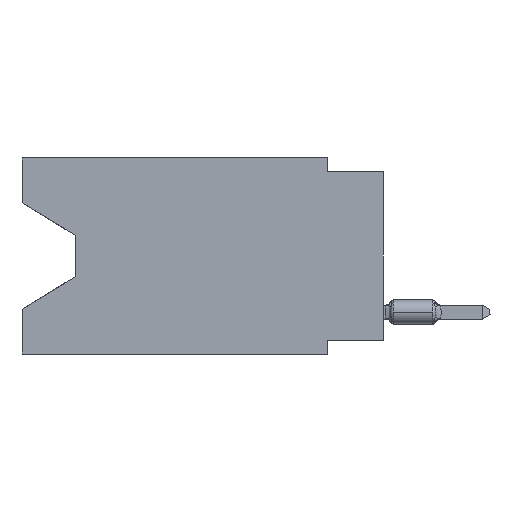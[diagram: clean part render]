
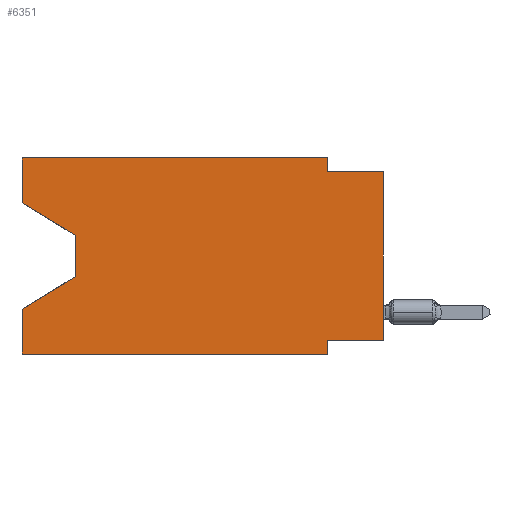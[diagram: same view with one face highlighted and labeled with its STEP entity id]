
A CAD part, left-side view. The second image highlights one B-rep face of the part: STEP entity #6351.
In plain terms, the highlighted planar face has unit normal (-1, 0, 0).
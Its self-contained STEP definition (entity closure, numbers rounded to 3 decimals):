
#263 = ORIENTED_EDGE ( 'NONE', *, *, #25929, .F. ) ;
#275 = CARTESIAN_POINT ( 'NONE',  ( 0., 0., -0.635 ) ) ;
#496 = ORIENTED_EDGE ( 'NONE', *, *, #4516, .T. ) ;
#847 = DIRECTION ( 'NONE',  ( 0., 0., -1. ) ) ;
#1204 = VERTEX_POINT ( 'NONE', #7517 ) ;
#1398 = EDGE_CURVE ( 'NONE', #16538, #1204, #17957, .T. ) ;
#1582 = EDGE_CURVE ( 'NONE', #8693, #20321, #19300, .T. ) ;
#1732 = ORIENTED_EDGE ( 'NONE', *, *, #1398, .F. ) ;
#1994 = EDGE_CURVE ( 'NONE', #21715, #24187, #12815, .T. ) ;
#2340 = CARTESIAN_POINT ( 'NONE',  ( 0., 16.383, 0. ) ) ;
#2963 = VECTOR ( 'NONE', #21807, 1000. ) ;
#3380 = VECTOR ( 'NONE', #6443, 1000. ) ;
#3395 = ORIENTED_EDGE ( 'NONE', *, *, #23280, .T. ) ;
#3563 = VECTOR ( 'NONE', #15848, 1000. ) ;
#3915 = VERTEX_POINT ( 'NONE', #27384 ) ;
#4516 = EDGE_CURVE ( 'NONE', #3915, #8952, #26525, .T. ) ;
#4691 = VECTOR ( 'NONE', #10370, 1000. ) ;
#4706 = VECTOR ( 'NONE', #27392, 1000. ) ;
#4714 = CARTESIAN_POINT ( 'NONE',  ( 0., 16.383, -6.852 ) ) ;
#5700 = ORIENTED_EDGE ( 'NONE', *, *, #8564, .F. ) ;
#5743 = EDGE_CURVE ( 'NONE', #1204, #20321, #18812, .T. ) ;
#6062 = DIRECTION ( 'NONE',  ( 1., 0., 0. ) ) ;
#6351 = ADVANCED_FACE ( 'NONE', ( #15439 ), #19857, .F. ) ;
#6443 = DIRECTION ( 'NONE',  ( 0., 1., 0. ) ) ;
#7517 = CARTESIAN_POINT ( 'NONE',  ( 0., 2.54, -8.255 ) ) ;
#8228 = CARTESIAN_POINT ( 'NONE',  ( 0., 0., -8.255 ) ) ;
#8269 = CARTESIAN_POINT ( 'NONE',  ( 0., 0., 0. ) ) ;
#8350 = VECTOR ( 'NONE', #9043, 1000. ) ;
#8355 = AXIS2_PLACEMENT_3D ( 'NONE', #26865, #6062, #24577 ) ;
#8564 = EDGE_CURVE ( 'NONE', #25387, #21715, #9311, .T. ) ;
#8693 = VERTEX_POINT ( 'NONE', #10201 ) ;
#8952 = VERTEX_POINT ( 'NONE', #4714 ) ;
#9043 = DIRECTION ( 'NONE',  ( 0., 0., 1. ) ) ;
#9311 = LINE ( 'NONE', #2340, #18099 ) ;
#9506 = EDGE_LOOP ( 'NONE', ( #15911, #26734, #496, #13155, #10331, #20762, #1732, #3395, #263, #22892, #5700, #11756 ) ) ;
#9807 = CARTESIAN_POINT ( 'NONE',  ( 0., 2.54, -0.635 ) ) ;
#10201 = CARTESIAN_POINT ( 'NONE',  ( 0., 16.383, -8.89 ) ) ;
#10331 = ORIENTED_EDGE ( 'NONE', *, *, #1582, .T. ) ;
#10370 = DIRECTION ( 'NONE',  ( 0., -1., 0. ) ) ;
#10612 = CARTESIAN_POINT ( 'NONE',  ( 0., 16.383, 0. ) ) ;
#11756 = ORIENTED_EDGE ( 'NONE', *, *, #21087, .F. ) ;
#11885 = DIRECTION ( 'NONE',  ( 0., -1., 0. ) ) ;
#12815 = LINE ( 'NONE', #14770, #13560 ) ;
#13155 = ORIENTED_EDGE ( 'NONE', *, *, #20713, .F. ) ;
#13560 = VECTOR ( 'NONE', #847, 1000. ) ;
#13596 = DIRECTION ( 'NONE',  ( 0., -0.855, -0.519 ) ) ;
#14584 = LINE ( 'NONE', #16158, #3563 ) ;
#14770 = CARTESIAN_POINT ( 'NONE',  ( 0., 2.54, 0. ) ) ;
#15439 = FACE_OUTER_BOUND ( 'NONE', #9506, .T. ) ;
#15523 = LINE ( 'NONE', #8269, #4706 ) ;
#15577 = CARTESIAN_POINT ( 'NONE',  ( 0., 16.383, -2.038 ) ) ;
#15592 = LINE ( 'NONE', #10612, #22390 ) ;
#15848 = DIRECTION ( 'NONE',  ( 0., 0., -1. ) ) ;
#15911 = ORIENTED_EDGE ( 'NONE', *, *, #28108, .T. ) ;
#16000 = CARTESIAN_POINT ( 'NONE',  ( 0., 16.383, 0. ) ) ;
#16158 = CARTESIAN_POINT ( 'NONE',  ( 0., 13.97, -3.505 ) ) ;
#16538 = VERTEX_POINT ( 'NONE', #8228 ) ;
#16712 = CARTESIAN_POINT ( 'NONE',  ( 0., 2.54, 0. ) ) ;
#16724 = CARTESIAN_POINT ( 'NONE',  ( 0., 16.383, -8.89 ) ) ;
#17957 = LINE ( 'NONE', #28926, #3380 ) ;
#18099 = VECTOR ( 'NONE', #29952, 1000. ) ;
#18812 = LINE ( 'NONE', #21244, #29157 ) ;
#18866 = VERTEX_POINT ( 'NONE', #21988 ) ;
#19300 = LINE ( 'NONE', #16724, #22743 ) ;
#19373 = CARTESIAN_POINT ( 'NONE',  ( 0., 13.97, -5.385 ) ) ;
#19857 = PLANE ( 'NONE',  #8355 ) ;
#20321 = VERTEX_POINT ( 'NONE', #23479 ) ;
#20713 = EDGE_CURVE ( 'NONE', #8693, #8952, #27564, .T. ) ;
#20762 = ORIENTED_EDGE ( 'NONE', *, *, #5743, .F. ) ;
#21024 = CARTESIAN_POINT ( 'NONE',  ( 0., 16.383, 0. ) ) ;
#21087 = EDGE_CURVE ( 'NONE', #18866, #25387, #15592, .T. ) ;
#21244 = CARTESIAN_POINT ( 'NONE',  ( 0., 2.54, -8.89 ) ) ;
#21646 = EDGE_CURVE ( 'NONE', #24533, #3915, #14584, .T. ) ;
#21715 = VERTEX_POINT ( 'NONE', #16712 ) ;
#21807 = DIRECTION ( 'NONE',  ( 0., 0.855, -0.519 ) ) ;
#21988 = CARTESIAN_POINT ( 'NONE',  ( 0., 16.383, -2.038 ) ) ;
#22390 = VECTOR ( 'NONE', #25162, 1000. ) ;
#22743 = VECTOR ( 'NONE', #11885, 1000. ) ;
#22892 = ORIENTED_EDGE ( 'NONE', *, *, #1994, .F. ) ;
#23280 = EDGE_CURVE ( 'NONE', #16538, #29787, #15523, .T. ) ;
#23479 = CARTESIAN_POINT ( 'NONE',  ( 0., 2.54, -8.89 ) ) ;
#24011 = LINE ( 'NONE', #26455, #4691 ) ;
#24187 = VERTEX_POINT ( 'NONE', #9807 ) ;
#24533 = VERTEX_POINT ( 'NONE', #27542 ) ;
#24577 = DIRECTION ( 'NONE',  ( 0., 0., -1. ) ) ;
#25162 = DIRECTION ( 'NONE',  ( 0., 0., 1. ) ) ;
#25387 = VERTEX_POINT ( 'NONE', #21024 ) ;
#25929 = EDGE_CURVE ( 'NONE', #24187, #29787, #24011, .T. ) ;
#26455 = CARTESIAN_POINT ( 'NONE',  ( 0., 0., -0.635 ) ) ;
#26525 = LINE ( 'NONE', #19373, #2963 ) ;
#26734 = ORIENTED_EDGE ( 'NONE', *, *, #21646, .T. ) ;
#26865 = CARTESIAN_POINT ( 'NONE',  ( 0., 16.383, 0. ) ) ;
#26995 = LINE ( 'NONE', #15577, #28188 ) ;
#27384 = CARTESIAN_POINT ( 'NONE',  ( 0., 13.97, -5.385 ) ) ;
#27392 = DIRECTION ( 'NONE',  ( 0., 0., 1. ) ) ;
#27542 = CARTESIAN_POINT ( 'NONE',  ( 0., 13.97, -3.505 ) ) ;
#27564 = LINE ( 'NONE', #16000, #8350 ) ;
#28089 = DIRECTION ( 'NONE',  ( 0., 0., -1. ) ) ;
#28108 = EDGE_CURVE ( 'NONE', #18866, #24533, #26995, .T. ) ;
#28188 = VECTOR ( 'NONE', #13596, 1000. ) ;
#28926 = CARTESIAN_POINT ( 'NONE',  ( 0., 0., -8.255 ) ) ;
#29157 = VECTOR ( 'NONE', #28089, 1000. ) ;
#29787 = VERTEX_POINT ( 'NONE', #275 ) ;
#29952 = DIRECTION ( 'NONE',  ( 0., -1., 0. ) ) ;
